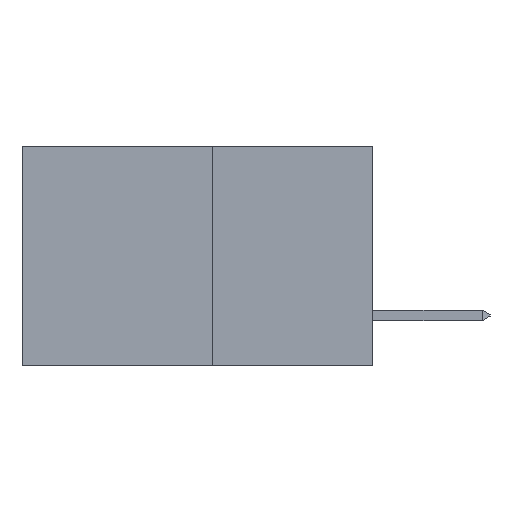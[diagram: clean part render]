
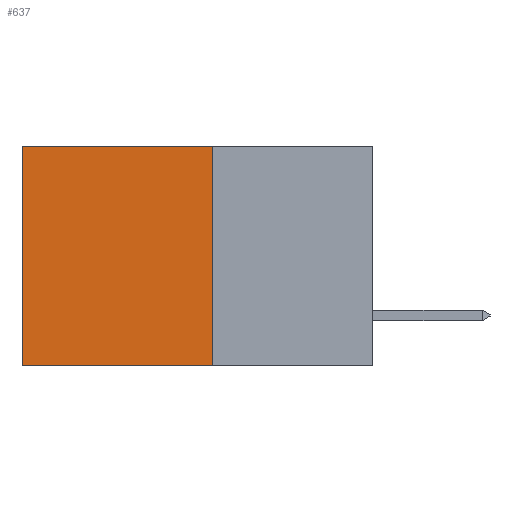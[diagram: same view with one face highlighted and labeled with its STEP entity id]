
A CAD part, left-side view. The second image highlights one B-rep face of the part: STEP entity #637.
In plain terms, the highlighted planar face has unit normal (-1, 0, 0).
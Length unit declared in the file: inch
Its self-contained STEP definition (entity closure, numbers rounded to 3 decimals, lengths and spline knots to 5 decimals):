
#64 = CARTESIAN_POINT ( 'NONE',  ( 0.277, 0.27, -0.37 ) ) ;
#218 = VERTEX_POINT ( 'NONE', #2662 ) ;
#636 = EDGE_CURVE ( 'NONE', #4598, #681, #1311, .T. ) ;
#637 = ADVANCED_FACE ( 'NONE', ( #791 ), #7479, .F. ) ;
#681 = VERTEX_POINT ( 'NONE', #5389 ) ;
#791 = FACE_OUTER_BOUND ( 'NONE', #8015, .T. ) ;
#856 = ORIENTED_EDGE ( 'NONE', *, *, #1186, .T. ) ;
#929 = AXIS2_PLACEMENT_3D ( 'NONE', #9306, #5361, #5640 ) ;
#1186 = EDGE_CURVE ( 'NONE', #218, #10224, #5984, .T. ) ;
#1311 = LINE ( 'NONE', #5758, #9260 ) ;
#1427 = DIRECTION ( 'NONE',  ( 0., 1., 0. ) ) ;
#2215 = LINE ( 'NONE', #3931, #4398 ) ;
#2282 = ORIENTED_EDGE ( 'NONE', *, *, #3770, .F. ) ;
#2423 = DIRECTION ( 'NONE',  ( 0., 0., -1. ) ) ;
#2465 = ORIENTED_EDGE ( 'NONE', *, *, #636, .F. ) ;
#2662 = CARTESIAN_POINT ( 'NONE',  ( 0.277, 0.59, 0. ) ) ;
#3151 = ORIENTED_EDGE ( 'NONE', *, *, #4397, .T. ) ;
#3770 = EDGE_CURVE ( 'NONE', #681, #10224, #7901, .T. ) ;
#3931 = CARTESIAN_POINT ( 'NONE',  ( 0.277, 0.27, 0. ) ) ;
#4032 = DIRECTION ( 'NONE',  ( 0., 0., -1. ) ) ;
#4142 = VECTOR ( 'NONE', #4032, 39.37008 ) ;
#4397 = EDGE_CURVE ( 'NONE', #4598, #218, #2215, .T. ) ;
#4398 = VECTOR ( 'NONE', #4976, 39.37008 ) ;
#4598 = VERTEX_POINT ( 'NONE', #7549 ) ;
#4976 = DIRECTION ( 'NONE',  ( 0., 1., 0. ) ) ;
#5361 = DIRECTION ( 'NONE',  ( 1., 0., 0. ) ) ;
#5389 = CARTESIAN_POINT ( 'NONE',  ( 0.277, 0.27, -0.37 ) ) ;
#5640 = DIRECTION ( 'NONE',  ( 0., 0., -1. ) ) ;
#5758 = CARTESIAN_POINT ( 'NONE',  ( 0.277, 0.27, -0.37 ) ) ;
#5984 = LINE ( 'NONE', #6194, #4142 ) ;
#6194 = CARTESIAN_POINT ( 'NONE',  ( 0.277, 0.59, -0.37 ) ) ;
#7479 = PLANE ( 'NONE',  #929 ) ;
#7549 = CARTESIAN_POINT ( 'NONE',  ( 0.277, 0.27, 0. ) ) ;
#7901 = LINE ( 'NONE', #64, #9738 ) ;
#8015 = EDGE_LOOP ( 'NONE', ( #856, #2282, #2465, #3151 ) ) ;
#9260 = VECTOR ( 'NONE', #2423, 39.37008 ) ;
#9306 = CARTESIAN_POINT ( 'NONE',  ( 0.277, 0.27, -0.37 ) ) ;
#9738 = VECTOR ( 'NONE', #1427, 39.37008 ) ;
#10224 = VERTEX_POINT ( 'NONE', #10231 ) ;
#10231 = CARTESIAN_POINT ( 'NONE',  ( 0.277, 0.59, -0.37 ) ) ;
